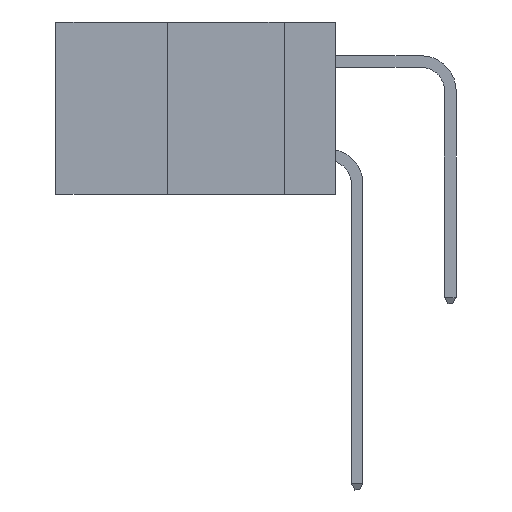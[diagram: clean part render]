
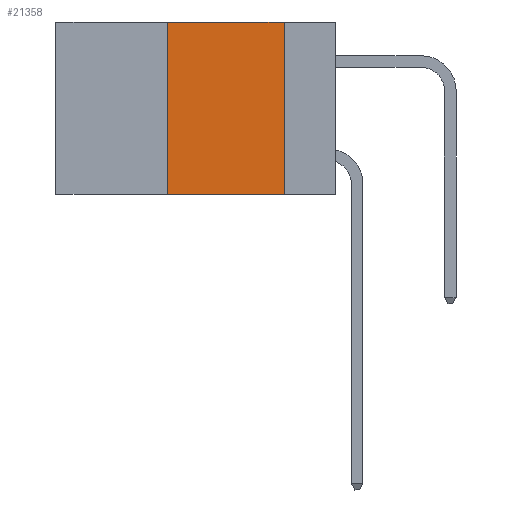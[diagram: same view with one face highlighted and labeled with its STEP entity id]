
A CAD part, left-side view. The second image highlights one B-rep face of the part: STEP entity #21358.
In plain terms, the highlighted planar face has unit normal (-1, 0, 0).
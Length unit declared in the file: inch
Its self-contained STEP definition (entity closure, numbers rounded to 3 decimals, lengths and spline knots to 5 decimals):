
#413 = DIRECTION ( 'NONE',  ( 1., 0., 0. ) ) ;
#3405 = CARTESIAN_POINT ( 'NONE',  ( 0., 0.11, 0. ) ) ;
#3858 = CARTESIAN_POINT ( 'NONE',  ( 0., 0.6, 0. ) ) ;
#5173 = CARTESIAN_POINT ( 'NONE',  ( 0., 0.11, 0. ) ) ;
#5769 = PLANE ( 'NONE',  #9326 ) ;
#6087 = VECTOR ( 'NONE', #8235, 39.37008 ) ;
#6248 = EDGE_CURVE ( 'NONE', #19352, #17292, #10672, .T. ) ;
#6290 = EDGE_CURVE ( 'NONE', #9370, #17292, #18468, .T. ) ;
#6354 = CARTESIAN_POINT ( 'NONE',  ( 0., 0.11, -0.37 ) ) ;
#6658 = CARTESIAN_POINT ( 'NONE',  ( 0., 0.6, 0. ) ) ;
#6730 = ORIENTED_EDGE ( 'NONE', *, *, #6290, .T. ) ;
#7832 = DIRECTION ( 'NONE',  ( 0., 0., 1. ) ) ;
#8235 = DIRECTION ( 'NONE',  ( 0., 0., -1. ) ) ;
#9326 = AXIS2_PLACEMENT_3D ( 'NONE', #3858, #413, #21241 ) ;
#9370 = VERTEX_POINT ( 'NONE', #14953 ) ;
#9958 = VECTOR ( 'NONE', #20474, 39.37008 ) ;
#10672 = LINE ( 'NONE', #5173, #6087 ) ;
#11777 = VERTEX_POINT ( 'NONE', #12343 ) ;
#12300 = DIRECTION ( 'NONE',  ( 0., -1., 0. ) ) ;
#12343 = CARTESIAN_POINT ( 'NONE',  ( 0., 0.36, 0. ) ) ;
#12576 = LINE ( 'NONE', #18155, #16635 ) ;
#13415 = ORIENTED_EDGE ( 'NONE', *, *, #15294, .F. ) ;
#13540 = EDGE_CURVE ( 'NONE', #11777, #19352, #20740, .T. ) ;
#14953 = CARTESIAN_POINT ( 'NONE',  ( 0., 0.36, -0.37 ) ) ;
#15294 = EDGE_CURVE ( 'NONE', #9370, #11777, #12576, .T. ) ;
#16635 = VECTOR ( 'NONE', #7832, 39.37008 ) ;
#17292 = VERTEX_POINT ( 'NONE', #6354 ) ;
#17897 = ORIENTED_EDGE ( 'NONE', *, *, #13540, .F. ) ;
#18155 = CARTESIAN_POINT ( 'NONE',  ( 0., 0.36, 0. ) ) ;
#18468 = LINE ( 'NONE', #20883, #21950 ) ;
#18534 = ORIENTED_EDGE ( 'NONE', *, *, #6248, .F. ) ;
#19130 = FACE_OUTER_BOUND ( 'NONE', #19460, .T. ) ;
#19352 = VERTEX_POINT ( 'NONE', #3405 ) ;
#19460 = EDGE_LOOP ( 'NONE', ( #18534, #17897, #13415, #6730 ) ) ;
#20474 = DIRECTION ( 'NONE',  ( 0., -1., 0. ) ) ;
#20740 = LINE ( 'NONE', #6658, #9958 ) ;
#20883 = CARTESIAN_POINT ( 'NONE',  ( 0., 0.6, -0.37 ) ) ;
#21241 = DIRECTION ( 'NONE',  ( 0., 0., -1. ) ) ;
#21358 = ADVANCED_FACE ( 'NONE', ( #19130 ), #5769, .F. ) ;
#21950 = VECTOR ( 'NONE', #12300, 39.37008 ) ;
